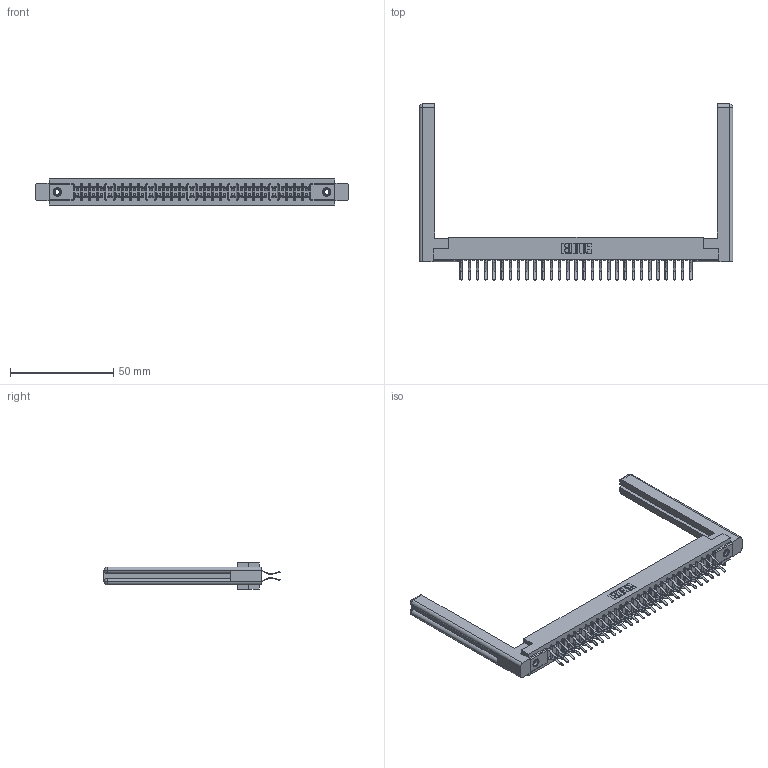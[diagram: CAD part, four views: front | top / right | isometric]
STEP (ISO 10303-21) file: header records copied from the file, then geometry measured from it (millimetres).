
FILE_DESCRIPTION (( 'STEP AP203' ), '1' );
FILE_NAME ('307-058-560-258.STEP', '2019-09-06T14:43:20', ( '' ), ( '' ), 'SwSTEP 2.0', 'SolidWorks 2016', '' );
FILE_SCHEMA (( 'CONFIG_CONTROL_DESIGN' ));
Length unit declared in the file: inch
Products named in the file (5): 307-220-058; 307 Part_.156 Dia Mounting Holes; 307-058-560-258; 307-290-001_560; 345-250-001_345-250-001-102
Assembly tree (63 placements, depth 2):
  307-058-560-258
    307 Part_.156 Dia Mounting Holes
    307-290-001_560  x58
    307-220-058  x2
    345-250-001_345-250-001-102  x2
Bounding box: 151.54 x 85.04 x 12.7 mm (x, y, z)
Volume: 23223.7 mm3; surface area: 24712.6 mm2
Topology: 63 solids, 63 shells, 3190 faces, 8913 edges, 5770 vertices
Faces by surface type: plane 2068, cylinder 1038, sphere 60, torus 12, cone 12
Entity records: 30129 total; most frequent: CARTESIAN_POINT 4952, ORIENTED_EDGE 4848, DIRECTION 4814, EDGE_CURVE 2424, VECTOR 1850, LINE 1850, VERTEX_POINT 1566, AXIS2_PLACEMENT_3D 1482
